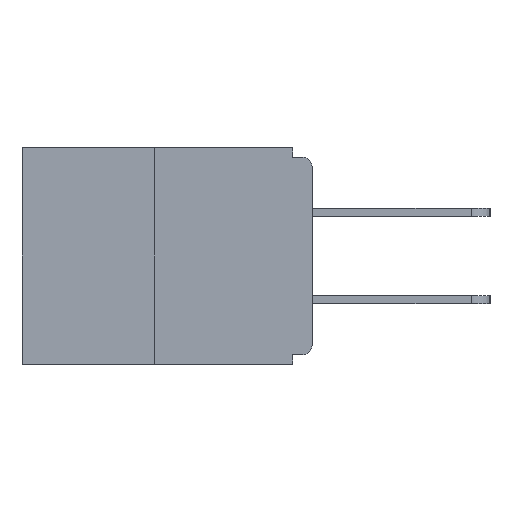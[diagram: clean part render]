
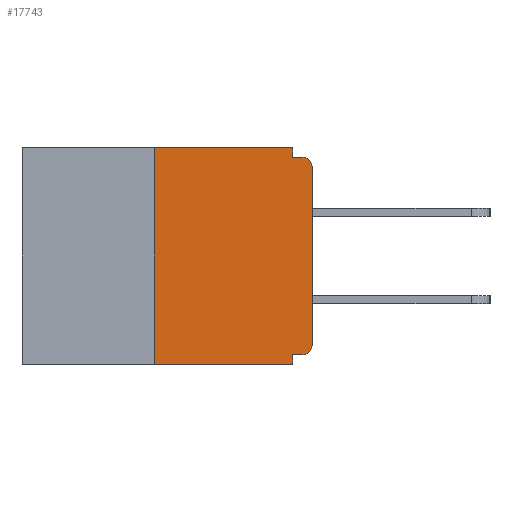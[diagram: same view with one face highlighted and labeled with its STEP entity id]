
A CAD part, left-side view. The second image highlights one B-rep face of the part: STEP entity #17743.
In plain terms, the highlighted planar face has unit normal (-1, 0, 0).
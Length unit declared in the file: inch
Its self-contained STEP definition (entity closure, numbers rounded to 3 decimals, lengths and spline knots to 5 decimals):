
#17 = CARTESIAN_POINT ( 'NONE',  ( 0., 0.25, -0.343 ) ) ;
#152 = ORIENTED_EDGE ( 'NONE', *, *, #19438, .T. ) ;
#901 = VECTOR ( 'NONE', #13988, 39.37008 ) ;
#909 = DIRECTION ( 'NONE',  ( -1., 0., 0. ) ) ;
#1031 = DIRECTION ( 'NONE',  ( 0., 1., 0. ) ) ;
#1619 = ORIENTED_EDGE ( 'NONE', *, *, #8531, .F. ) ;
#1784 = FACE_OUTER_BOUND ( 'NONE', #8576, .T. ) ;
#1881 = CARTESIAN_POINT ( 'NONE',  ( 0., 0., -0.313 ) ) ;
#1897 = ORIENTED_EDGE ( 'NONE', *, *, #16240, .F. ) ;
#1926 = AXIS2_PLACEMENT_3D ( 'NONE', #19383, #8238, #3248 ) ;
#2180 = CARTESIAN_POINT ( 'NONE',  ( 0., 0.25, 0. ) ) ;
#2231 = LINE ( 'NONE', #19017, #12870 ) ;
#2635 = VECTOR ( 'NONE', #1031, 39.37008 ) ;
#3039 = EDGE_CURVE ( 'NONE', #3244, #17171, #19785, .T. ) ;
#3238 = CARTESIAN_POINT ( 'NONE',  ( 0., 0.031, 0. ) ) ;
#3244 = VERTEX_POINT ( 'NONE', #3238 ) ;
#3248 = DIRECTION ( 'NONE',  ( 0., 0., -1. ) ) ;
#4168 = DIRECTION ( 'NONE',  ( 0., -1., 0. ) ) ;
#4237 = ORIENTED_EDGE ( 'NONE', *, *, #13557, .F. ) ;
#4547 = CIRCLE ( 'NONE', #1926, 0.015 ) ;
#4882 = CARTESIAN_POINT ( 'NONE',  ( 0., 0.015, -0.328 ) ) ;
#5036 = DIRECTION ( 'NONE',  ( 1., 0., 0. ) ) ;
#5412 = LINE ( 'NONE', #7418, #2635 ) ;
#5542 = CARTESIAN_POINT ( 'NONE',  ( 0., 0.015, -0.03 ) ) ;
#6230 = DIRECTION ( 'NONE',  ( 0., 0., -1. ) ) ;
#6427 = CARTESIAN_POINT ( 'NONE',  ( 0., 0.031, -0.343 ) ) ;
#6461 = VERTEX_POINT ( 'NONE', #20071 ) ;
#6668 = CARTESIAN_POINT ( 'NONE',  ( 0., 0.015, -0.015 ) ) ;
#7283 = ORIENTED_EDGE ( 'NONE', *, *, #18369, .T. ) ;
#7294 = DIRECTION ( 'NONE',  ( 0., 0., -1. ) ) ;
#7418 = CARTESIAN_POINT ( 'NONE',  ( 0., 0., -0.328 ) ) ;
#8004 = EDGE_CURVE ( 'NONE', #8328, #15088, #19842, .T. ) ;
#8238 = DIRECTION ( 'NONE',  ( -1., 0., 0. ) ) ;
#8328 = VERTEX_POINT ( 'NONE', #17 ) ;
#8530 = DIRECTION ( 'NONE',  ( 0., -1., 0. ) ) ;
#8531 = EDGE_CURVE ( 'NONE', #8328, #16384, #11003, .T. ) ;
#8576 = EDGE_LOOP ( 'NONE', ( #17262, #1619, #14028, #1897, #11741, #7283, #16401, #152, #4237, #11405 ) ) ;
#8649 = AXIS2_PLACEMENT_3D ( 'NONE', #16305, #5036, #14964 ) ;
#10146 = LINE ( 'NONE', #12626, #13950 ) ;
#10181 = CARTESIAN_POINT ( 'NONE',  ( 0., 0.031, -0.343 ) ) ;
#10462 = EDGE_CURVE ( 'NONE', #19427, #6461, #10146, .T. ) ;
#10656 = CARTESIAN_POINT ( 'NONE',  ( 0., 0.25, 0. ) ) ;
#10927 = DIRECTION ( 'NONE',  ( 0., 0., 1. ) ) ;
#11003 = LINE ( 'NONE', #10656, #901 ) ;
#11405 = ORIENTED_EDGE ( 'NONE', *, *, #3039, .F. ) ;
#11535 = CARTESIAN_POINT ( 'NONE',  ( 0., 0.031, -0.015 ) ) ;
#11741 = ORIENTED_EDGE ( 'NONE', *, *, #14753, .F. ) ;
#11775 = VECTOR ( 'NONE', #8530, 39.37008 ) ;
#11878 = EDGE_CURVE ( 'NONE', #16384, #3244, #2231, .T. ) ;
#12032 = DIRECTION ( 'NONE',  ( 0., -1., 0. ) ) ;
#12202 = VERTEX_POINT ( 'NONE', #6668 ) ;
#12626 = CARTESIAN_POINT ( 'NONE',  ( 0., 0., 0. ) ) ;
#12870 = VECTOR ( 'NONE', #4168, 39.37008 ) ;
#12969 = PLANE ( 'NONE',  #8649 ) ;
#13202 = VECTOR ( 'NONE', #6230, 39.37008 ) ;
#13303 = CARTESIAN_POINT ( 'NONE',  ( 0., 0.46, -0.343 ) ) ;
#13557 = EDGE_CURVE ( 'NONE', #17171, #12202, #17845, .T. ) ;
#13950 = VECTOR ( 'NONE', #10927, 39.37008 ) ;
#13988 = DIRECTION ( 'NONE',  ( 0., 0., 1. ) ) ;
#14028 = ORIENTED_EDGE ( 'NONE', *, *, #8004, .T. ) ;
#14753 = EDGE_CURVE ( 'NONE', #16900, #17618, #5412, .T. ) ;
#14964 = DIRECTION ( 'NONE',  ( 0., 0., -1. ) ) ;
#15021 = VECTOR ( 'NONE', #15915, 39.37008 ) ;
#15088 = VERTEX_POINT ( 'NONE', #10181 ) ;
#15278 = LINE ( 'NONE', #6427, #15021 ) ;
#15285 = VECTOR ( 'NONE', #12032, 39.37008 ) ;
#15617 = CIRCLE ( 'NONE', #20226, 0.015 ) ;
#15915 = DIRECTION ( 'NONE',  ( 0., 0., -1. ) ) ;
#16240 = EDGE_CURVE ( 'NONE', #17618, #15088, #15278, .T. ) ;
#16305 = CARTESIAN_POINT ( 'NONE',  ( 0., 0.46, 0. ) ) ;
#16384 = VERTEX_POINT ( 'NONE', #2180 ) ;
#16401 = ORIENTED_EDGE ( 'NONE', *, *, #10462, .T. ) ;
#16495 = CARTESIAN_POINT ( 'NONE',  ( 0., 0., -0.015 ) ) ;
#16900 = VERTEX_POINT ( 'NONE', #4882 ) ;
#17171 = VERTEX_POINT ( 'NONE', #11535 ) ;
#17262 = ORIENTED_EDGE ( 'NONE', *, *, #11878, .F. ) ;
#17618 = VERTEX_POINT ( 'NONE', #19068 ) ;
#17743 = ADVANCED_FACE ( 'NONE', ( #1784 ), #12969, .F. ) ;
#17845 = LINE ( 'NONE', #16495, #15285 ) ;
#18369 = EDGE_CURVE ( 'NONE', #16900, #19427, #4547, .T. ) ;
#19017 = CARTESIAN_POINT ( 'NONE',  ( 0., 0.46, 0. ) ) ;
#19068 = CARTESIAN_POINT ( 'NONE',  ( 0., 0.031, -0.328 ) ) ;
#19383 = CARTESIAN_POINT ( 'NONE',  ( 0., 0.015, -0.313 ) ) ;
#19427 = VERTEX_POINT ( 'NONE', #1881 ) ;
#19438 = EDGE_CURVE ( 'NONE', #6461, #12202, #15617, .T. ) ;
#19785 = LINE ( 'NONE', #20725, #13202 ) ;
#19842 = LINE ( 'NONE', #13303, #11775 ) ;
#20071 = CARTESIAN_POINT ( 'NONE',  ( 0., 0., -0.03 ) ) ;
#20226 = AXIS2_PLACEMENT_3D ( 'NONE', #5542, #909, #7294 ) ;
#20725 = CARTESIAN_POINT ( 'NONE',  ( 0., 0.031, 0. ) ) ;
